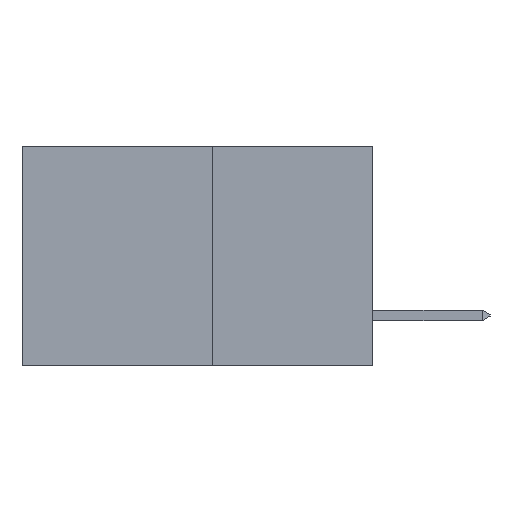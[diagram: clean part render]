
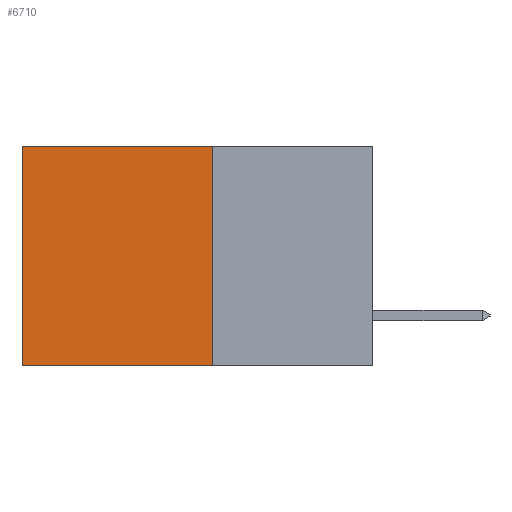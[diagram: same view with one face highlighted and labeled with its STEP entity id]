
A CAD part, left-side view. The second image highlights one B-rep face of the part: STEP entity #6710.
In plain terms, the highlighted planar face has unit normal (-1, 0, 0).
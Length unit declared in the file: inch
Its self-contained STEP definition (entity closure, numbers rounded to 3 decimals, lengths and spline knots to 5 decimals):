
#606 = PLANE ( 'NONE',  #18069 ) ;
#681 = DIRECTION ( 'NONE',  ( 0., 1., 0. ) ) ;
#1311 = DIRECTION ( 'NONE',  ( 1., 0., 0. ) ) ;
#1605 = VERTEX_POINT ( 'NONE', #6381 ) ;
#1762 = CARTESIAN_POINT ( 'NONE',  ( 0.277, 0.27, 0. ) ) ;
#2188 = CARTESIAN_POINT ( 'NONE',  ( 0.277, 0.27, -0.37 ) ) ;
#2241 = LINE ( 'NONE', #2188, #16492 ) ;
#2580 = DIRECTION ( 'NONE',  ( 0., 0., -1. ) ) ;
#2595 = CARTESIAN_POINT ( 'NONE',  ( 0.277, 0.59, -0.37 ) ) ;
#2620 = EDGE_CURVE ( 'NONE', #15062, #17266, #4136, .T. ) ;
#2681 = LINE ( 'NONE', #13637, #17305 ) ;
#4136 = LINE ( 'NONE', #12125, #5054 ) ;
#4186 = DIRECTION ( 'NONE',  ( 0., 1., 0. ) ) ;
#5054 = VECTOR ( 'NONE', #11439, 39.37008 ) ;
#5276 = EDGE_CURVE ( 'NONE', #1605, #15062, #7746, .T. ) ;
#5563 = CARTESIAN_POINT ( 'NONE',  ( 0.277, 0.59, 0. ) ) ;
#5589 = EDGE_CURVE ( 'NONE', #1605, #7141, #2681, .T. ) ;
#5632 = EDGE_CURVE ( 'NONE', #7141, #17266, #2241, .T. ) ;
#6381 = CARTESIAN_POINT ( 'NONE',  ( 0.277, 0.27, 0. ) ) ;
#6710 = ADVANCED_FACE ( 'NONE', ( #7232 ), #606, .F. ) ;
#7141 = VERTEX_POINT ( 'NONE', #8919 ) ;
#7232 = FACE_OUTER_BOUND ( 'NONE', #9219, .T. ) ;
#7746 = LINE ( 'NONE', #1762, #11145 ) ;
#8633 = ORIENTED_EDGE ( 'NONE', *, *, #5632, .F. ) ;
#8919 = CARTESIAN_POINT ( 'NONE',  ( 0.277, 0.27, -0.37 ) ) ;
#9219 = EDGE_LOOP ( 'NONE', ( #12372, #8633, #18305, #15803 ) ) ;
#9683 = DIRECTION ( 'NONE',  ( 0., 0., -1. ) ) ;
#11145 = VECTOR ( 'NONE', #4186, 39.37008 ) ;
#11439 = DIRECTION ( 'NONE',  ( 0., 0., -1. ) ) ;
#12125 = CARTESIAN_POINT ( 'NONE',  ( 0.277, 0.59, -0.37 ) ) ;
#12372 = ORIENTED_EDGE ( 'NONE', *, *, #2620, .T. ) ;
#13637 = CARTESIAN_POINT ( 'NONE',  ( 0.277, 0.27, -0.37 ) ) ;
#15062 = VERTEX_POINT ( 'NONE', #5563 ) ;
#15803 = ORIENTED_EDGE ( 'NONE', *, *, #5276, .T. ) ;
#15901 = CARTESIAN_POINT ( 'NONE',  ( 0.277, 0.27, -0.37 ) ) ;
#16492 = VECTOR ( 'NONE', #681, 39.37008 ) ;
#17266 = VERTEX_POINT ( 'NONE', #2595 ) ;
#17305 = VECTOR ( 'NONE', #2580, 39.37008 ) ;
#18069 = AXIS2_PLACEMENT_3D ( 'NONE', #15901, #1311, #9683 ) ;
#18305 = ORIENTED_EDGE ( 'NONE', *, *, #5589, .F. ) ;
